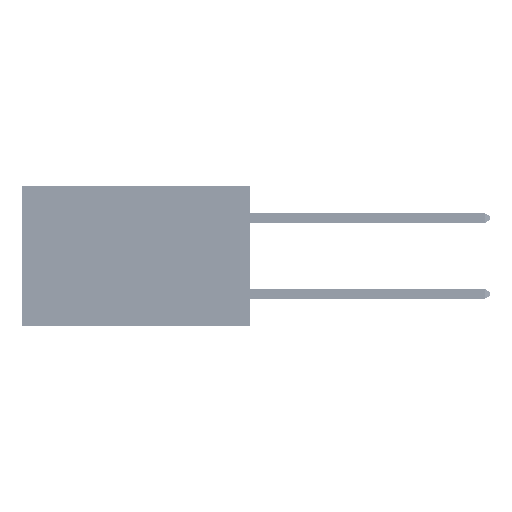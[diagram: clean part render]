
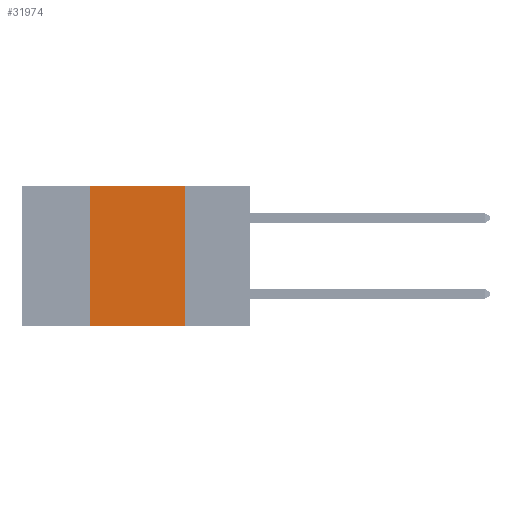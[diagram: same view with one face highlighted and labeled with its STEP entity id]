
A CAD part, left-side view. The second image highlights one B-rep face of the part: STEP entity #31974.
In plain terms, the highlighted planar face has unit normal (-1, 0, 0).
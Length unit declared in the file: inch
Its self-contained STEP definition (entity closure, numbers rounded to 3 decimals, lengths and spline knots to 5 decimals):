
#86 = EDGE_CURVE ( 'NONE', #36753, #41861, #13260, .T. ) ;
#1234 = LINE ( 'NONE', #43291, #49585 ) ;
#5503 = DIRECTION ( 'NONE',  ( 0., -1., 0. ) ) ;
#8278 = AXIS2_PLACEMENT_3D ( 'NONE', #32589, #40580, #12563 ) ;
#11089 = ORIENTED_EDGE ( 'NONE', *, *, #16307, .F. ) ;
#11253 = CARTESIAN_POINT ( 'NONE',  ( 0., 0.6, 0. ) ) ;
#12037 = DIRECTION ( 'NONE',  ( 0., 0., -1. ) ) ;
#12563 = DIRECTION ( 'NONE',  ( 0., 0., -1. ) ) ;
#13260 = LINE ( 'NONE', #14608, #39494 ) ;
#14608 = CARTESIAN_POINT ( 'NONE',  ( 0., 0.42, 0. ) ) ;
#14801 = CARTESIAN_POINT ( 'NONE',  ( 0., 0.17, 0. ) ) ;
#16307 = EDGE_CURVE ( 'NONE', #28792, #37210, #1234, .T. ) ;
#27006 = DIRECTION ( 'NONE',  ( 0., -1., 0. ) ) ;
#28792 = VERTEX_POINT ( 'NONE', #14801 ) ;
#28815 = PLANE ( 'NONE',  #8278 ) ;
#30919 = ORIENTED_EDGE ( 'NONE', *, *, #86, .F. ) ;
#31399 = CARTESIAN_POINT ( 'NONE',  ( 0., 0.6, -0.37 ) ) ;
#31974 = ADVANCED_FACE ( 'NONE', ( #34477 ), #28815, .F. ) ;
#32589 = CARTESIAN_POINT ( 'NONE',  ( 0., 0.6, 0. ) ) ;
#34477 = FACE_OUTER_BOUND ( 'NONE', #48555, .T. ) ;
#34752 = VECTOR ( 'NONE', #27006, 39.37008 ) ;
#35289 = CARTESIAN_POINT ( 'NONE',  ( 0., 0.42, 0. ) ) ;
#36753 = VERTEX_POINT ( 'NONE', #38499 ) ;
#37210 = VERTEX_POINT ( 'NONE', #44955 ) ;
#38130 = ORIENTED_EDGE ( 'NONE', *, *, #48885, .F. ) ;
#38499 = CARTESIAN_POINT ( 'NONE',  ( 0., 0.42, -0.37 ) ) ;
#38743 = ORIENTED_EDGE ( 'NONE', *, *, #39594, .T. ) ;
#38973 = VECTOR ( 'NONE', #5503, 39.37008 ) ;
#39494 = VECTOR ( 'NONE', #41905, 39.37008 ) ;
#39594 = EDGE_CURVE ( 'NONE', #36753, #37210, #49336, .T. ) ;
#39620 = LINE ( 'NONE', #11253, #34752 ) ;
#40580 = DIRECTION ( 'NONE',  ( 1., 0., 0. ) ) ;
#41861 = VERTEX_POINT ( 'NONE', #35289 ) ;
#41905 = DIRECTION ( 'NONE',  ( 0., 0., 1. ) ) ;
#43291 = CARTESIAN_POINT ( 'NONE',  ( 0., 0.17, 0. ) ) ;
#44955 = CARTESIAN_POINT ( 'NONE',  ( 0., 0.17, -0.37 ) ) ;
#48555 = EDGE_LOOP ( 'NONE', ( #11089, #38130, #30919, #38743 ) ) ;
#48885 = EDGE_CURVE ( 'NONE', #41861, #28792, #39620, .T. ) ;
#49336 = LINE ( 'NONE', #31399, #38973 ) ;
#49585 = VECTOR ( 'NONE', #12037, 39.37008 ) ;
